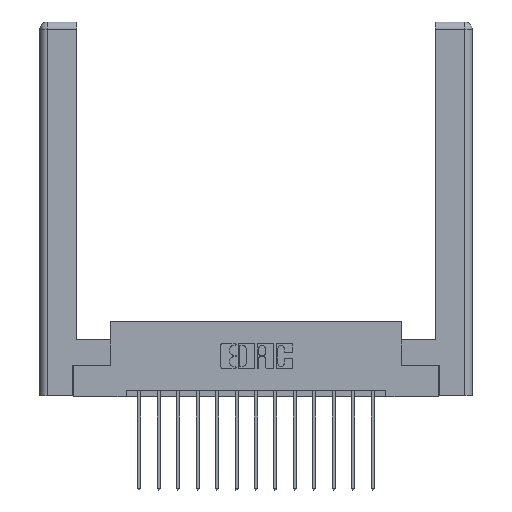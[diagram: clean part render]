
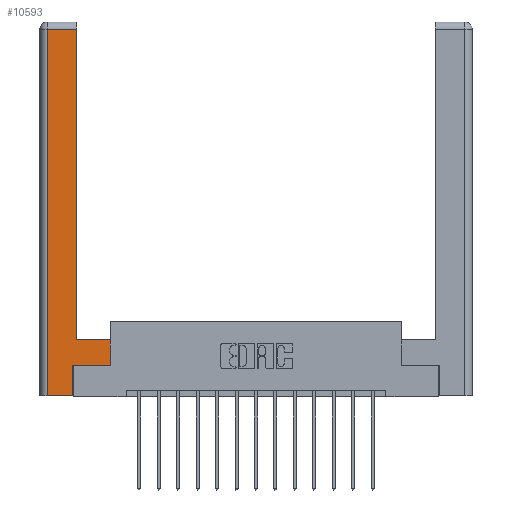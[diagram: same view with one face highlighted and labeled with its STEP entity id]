
A CAD part, top view. The second image highlights one B-rep face of the part: STEP entity #10593.
In plain terms, the highlighted planar face has unit normal (0, 0, 1).
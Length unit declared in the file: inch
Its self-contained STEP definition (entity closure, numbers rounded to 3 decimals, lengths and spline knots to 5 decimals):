
#20 = EDGE_CURVE ( 'NONE', #16459, #10477, #2092, .T. ) ;
#88 = LINE ( 'NONE', #2468, #3656 ) ;
#188 = DIRECTION ( 'NONE',  ( 0., 1., 0. ) ) ;
#550 = ORIENTED_EDGE ( 'NONE', *, *, #14650, .T. ) ;
#560 = LINE ( 'NONE', #3802, #2346 ) ;
#692 = ORIENTED_EDGE ( 'NONE', *, *, #5903, .T. ) ;
#1402 = FACE_OUTER_BOUND ( 'NONE', #2762, .T. ) ;
#1438 = CARTESIAN_POINT ( 'NONE',  ( 0.0615, 0., 0. ) ) ;
#1896 = VECTOR ( 'NONE', #13380, 39.37008 ) ;
#1972 = CARTESIAN_POINT ( 'NONE',  ( 0.0615, 0., 0. ) ) ;
#2076 = CARTESIAN_POINT ( 'NONE',  ( 0.565, 0.45, 0. ) ) ;
#2092 = LINE ( 'NONE', #12189, #1896 ) ;
#2290 = CARTESIAN_POINT ( 'NONE',  ( 0.295, 3., 0. ) ) ;
#2346 = VECTOR ( 'NONE', #12687, 39.37008 ) ;
#2468 = CARTESIAN_POINT ( 'NONE',  ( 0.265, 0., 0. ) ) ;
#2733 = ORIENTED_EDGE ( 'NONE', *, *, #13121, .T. ) ;
#2762 = EDGE_LOOP ( 'NONE', ( #11289, #6869, #2733, #5112, #692, #550, #9228, #9205 ) ) ;
#3477 = DIRECTION ( 'NONE',  ( 0., -1., 0. ) ) ;
#3656 = VECTOR ( 'NONE', #11739, 39.37008 ) ;
#3802 = CARTESIAN_POINT ( 'NONE',  ( 0.0615, 2.94, 0. ) ) ;
#4755 = PLANE ( 'NONE',  #8936 ) ;
#4757 = EDGE_CURVE ( 'NONE', #8182, #5747, #560, .T. ) ;
#5062 = EDGE_CURVE ( 'NONE', #14204, #16459, #11035, .T. ) ;
#5112 = ORIENTED_EDGE ( 'NONE', *, *, #14810, .T. ) ;
#5747 = VERTEX_POINT ( 'NONE', #11049 ) ;
#5903 = EDGE_CURVE ( 'NONE', #15992, #7455, #12757, .T. ) ;
#6419 = CARTESIAN_POINT ( 'NONE',  ( 0.565, 0.245, 0. ) ) ;
#6798 = CARTESIAN_POINT ( 'NONE',  ( 0.265, 0.245, 0. ) ) ;
#6869 = ORIENTED_EDGE ( 'NONE', *, *, #4757, .T. ) ;
#7455 = VERTEX_POINT ( 'NONE', #6798 ) ;
#8182 = VERTEX_POINT ( 'NONE', #15838 ) ;
#8653 = CARTESIAN_POINT ( 'NONE',  ( 0., 0., 0. ) ) ;
#8936 = AXIS2_PLACEMENT_3D ( 'NONE', #8653, #13713, #10177 ) ;
#9205 = ORIENTED_EDGE ( 'NONE', *, *, #20, .T. ) ;
#9228 = ORIENTED_EDGE ( 'NONE', *, *, #5062, .T. ) ;
#9887 = CARTESIAN_POINT ( 'NONE',  ( 0.565, 0.245, 0. ) ) ;
#10177 = DIRECTION ( 'NONE',  ( -1., 0., 0. ) ) ;
#10477 = VERTEX_POINT ( 'NONE', #15504 ) ;
#10593 = ADVANCED_FACE ( 'NONE', ( #1402 ), #4755, .F. ) ;
#10711 = VERTEX_POINT ( 'NONE', #1438 ) ;
#11035 = LINE ( 'NONE', #14490, #14046 ) ;
#11049 = CARTESIAN_POINT ( 'NONE',  ( 0.0615, 2.94, 0. ) ) ;
#11289 = ORIENTED_EDGE ( 'NONE', *, *, #11688, .T. ) ;
#11688 = EDGE_CURVE ( 'NONE', #10477, #8182, #15706, .T. ) ;
#11739 = DIRECTION ( 'NONE',  ( 1., 0., 0. ) ) ;
#11854 = DIRECTION ( 'NONE',  ( 0., 1., 0. ) ) ;
#12189 = CARTESIAN_POINT ( 'NONE',  ( 0.295, 0.45, 0. ) ) ;
#12524 = DIRECTION ( 'NONE',  ( 1., 0., 0. ) ) ;
#12647 = LINE ( 'NONE', #9887, #15827 ) ;
#12687 = DIRECTION ( 'NONE',  ( -1., 0., 0. ) ) ;
#12757 = LINE ( 'NONE', #15065, #15560 ) ;
#12887 = LINE ( 'NONE', #1972, #13897 ) ;
#13121 = EDGE_CURVE ( 'NONE', #5747, #10711, #12887, .T. ) ;
#13380 = DIRECTION ( 'NONE',  ( -1., 0., 0. ) ) ;
#13713 = DIRECTION ( 'NONE',  ( 0., 0., -1. ) ) ;
#13897 = VECTOR ( 'NONE', #3477, 39.37008 ) ;
#14046 = VECTOR ( 'NONE', #11854, 39.37008 ) ;
#14204 = VERTEX_POINT ( 'NONE', #6419 ) ;
#14490 = CARTESIAN_POINT ( 'NONE',  ( 0.565, 0.45, 0. ) ) ;
#14650 = EDGE_CURVE ( 'NONE', #7455, #14204, #12647, .T. ) ;
#14724 = VECTOR ( 'NONE', #15075, 39.37008 ) ;
#14810 = EDGE_CURVE ( 'NONE', #10711, #15992, #88, .T. ) ;
#15052 = CARTESIAN_POINT ( 'NONE',  ( 0.265, 0., 0. ) ) ;
#15065 = CARTESIAN_POINT ( 'NONE',  ( 0.265, 0.245, 0. ) ) ;
#15075 = DIRECTION ( 'NONE',  ( 0., 1., 0. ) ) ;
#15504 = CARTESIAN_POINT ( 'NONE',  ( 0.295, 0.45, 0. ) ) ;
#15560 = VECTOR ( 'NONE', #188, 39.37008 ) ;
#15706 = LINE ( 'NONE', #2290, #14724 ) ;
#15827 = VECTOR ( 'NONE', #12524, 39.37008 ) ;
#15838 = CARTESIAN_POINT ( 'NONE',  ( 0.295, 2.94, 0. ) ) ;
#15992 = VERTEX_POINT ( 'NONE', #15052 ) ;
#16459 = VERTEX_POINT ( 'NONE', #2076 ) ;
